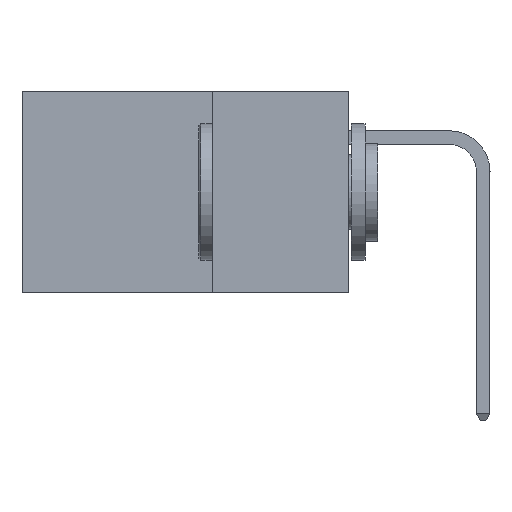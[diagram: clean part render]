
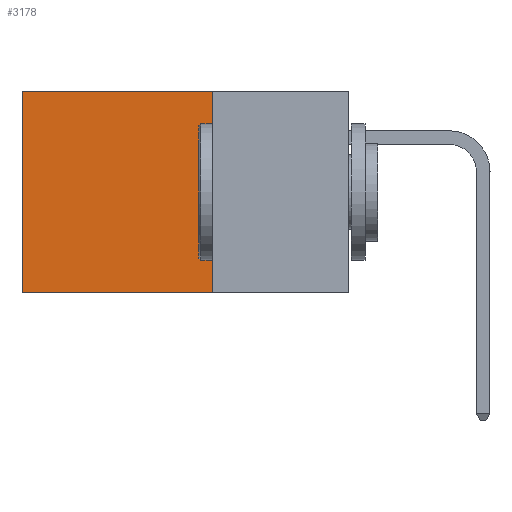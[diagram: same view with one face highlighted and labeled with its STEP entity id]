
A CAD part, left-side view. The second image highlights one B-rep face of the part: STEP entity #3178.
In plain terms, the highlighted planar face has unit normal (-1, 0, 0).
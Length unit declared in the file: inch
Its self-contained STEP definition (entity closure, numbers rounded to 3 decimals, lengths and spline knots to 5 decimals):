
#2340 = LINE ( 'NONE', #44645, #40118 ) ;
#2826 = ORIENTED_EDGE ( 'NONE', *, *, #5659, .T. ) ;
#3178 = ADVANCED_FACE ( 'NONE', ( #20394 ), #36027, .F. ) ;
#4868 = ORIENTED_EDGE ( 'NONE', *, *, #25042, .F. ) ;
#5659 = EDGE_CURVE ( 'NONE', #29872, #40264, #27376, .T. ) ;
#5774 = CARTESIAN_POINT ( 'NONE',  ( 0.2875, 0.6, -0.37 ) ) ;
#11305 = CARTESIAN_POINT ( 'NONE',  ( 0.2875, 0.25, 0. ) ) ;
#12529 = VERTEX_POINT ( 'NONE', #5774 ) ;
#14260 = ORIENTED_EDGE ( 'NONE', *, *, #41635, .F. ) ;
#17407 = DIRECTION ( 'NONE',  ( 0., 0., -1. ) ) ;
#18546 = DIRECTION ( 'NONE',  ( 0., 0., -1. ) ) ;
#20394 = FACE_OUTER_BOUND ( 'NONE', #20953, .T. ) ;
#20953 = EDGE_LOOP ( 'NONE', ( #38861, #4868, #14260, #2826 ) ) ;
#23681 = DIRECTION ( 'NONE',  ( 0., 1., 0. ) ) ;
#23971 = LINE ( 'NONE', #29807, #33318 ) ;
#25042 = EDGE_CURVE ( 'NONE', #39296, #12529, #2340, .T. ) ;
#27376 = LINE ( 'NONE', #35213, #44884 ) ;
#27608 = VECTOR ( 'NONE', #17407, 39.37008 ) ;
#28020 = LINE ( 'NONE', #38565, #27608 ) ;
#28321 = DIRECTION ( 'NONE',  ( 0., 1., 0. ) ) ;
#29807 = CARTESIAN_POINT ( 'NONE',  ( 0.2875, 0.6, 0. ) ) ;
#29872 = VERTEX_POINT ( 'NONE', #41993 ) ;
#30723 = CARTESIAN_POINT ( 'NONE',  ( 0.2875, 0.6, 0. ) ) ;
#31341 = AXIS2_PLACEMENT_3D ( 'NONE', #11305, #39532, #18546 ) ;
#33318 = VECTOR ( 'NONE', #36711, 39.37008 ) ;
#35213 = CARTESIAN_POINT ( 'NONE',  ( 0.2875, 0.25, 0. ) ) ;
#35408 = EDGE_CURVE ( 'NONE', #40264, #12529, #23971, .T. ) ;
#36027 = PLANE ( 'NONE',  #31341 ) ;
#36711 = DIRECTION ( 'NONE',  ( 0., 0., -1. ) ) ;
#38565 = CARTESIAN_POINT ( 'NONE',  ( 0.2875, 0.25, 0. ) ) ;
#38861 = ORIENTED_EDGE ( 'NONE', *, *, #35408, .T. ) ;
#39296 = VERTEX_POINT ( 'NONE', #45034 ) ;
#39532 = DIRECTION ( 'NONE',  ( 1., 0., 0. ) ) ;
#40118 = VECTOR ( 'NONE', #23681, 39.37008 ) ;
#40264 = VERTEX_POINT ( 'NONE', #30723 ) ;
#41635 = EDGE_CURVE ( 'NONE', #29872, #39296, #28020, .T. ) ;
#41993 = CARTESIAN_POINT ( 'NONE',  ( 0.2875, 0.25, 0. ) ) ;
#44645 = CARTESIAN_POINT ( 'NONE',  ( 0.2875, 0.25, -0.37 ) ) ;
#44884 = VECTOR ( 'NONE', #28321, 39.37008 ) ;
#45034 = CARTESIAN_POINT ( 'NONE',  ( 0.2875, 0.25, -0.37 ) ) ;
